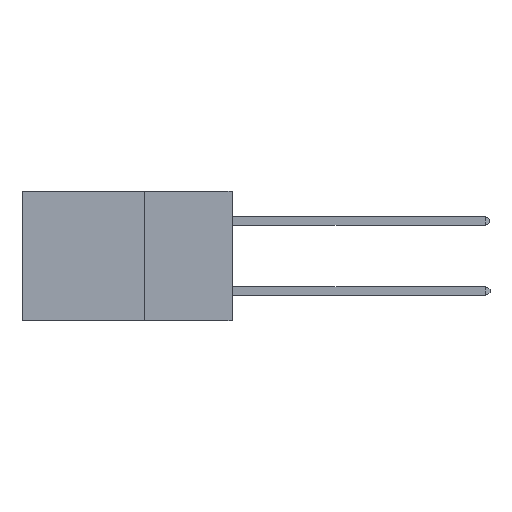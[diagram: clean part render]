
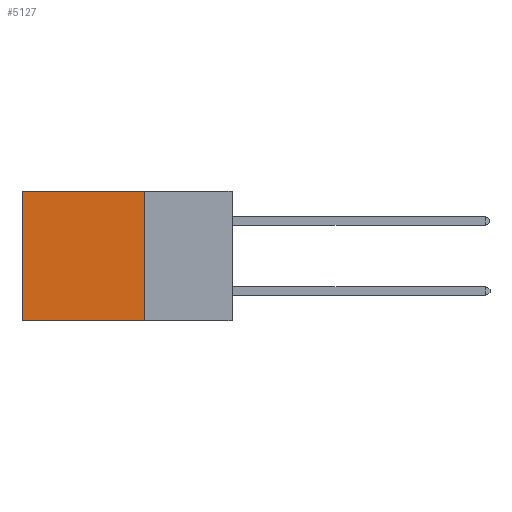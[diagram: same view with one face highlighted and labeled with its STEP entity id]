
A CAD part, left-side view. The second image highlights one B-rep face of the part: STEP entity #5127.
In plain terms, the highlighted planar face has unit normal (-1, 0, 0).
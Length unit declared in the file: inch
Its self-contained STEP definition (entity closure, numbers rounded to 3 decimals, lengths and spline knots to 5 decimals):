
#212 = EDGE_CURVE ( 'NONE', #12373, #5416, #5501, .T. ) ;
#460 = CARTESIAN_POINT ( 'NONE',  ( 0.2875, 0.6, -0.37 ) ) ;
#542 = FACE_OUTER_BOUND ( 'NONE', #8381, .T. ) ;
#836 = LINE ( 'NONE', #8320, #11488 ) ;
#1406 = VECTOR ( 'NONE', #11920, 39.37008 ) ;
#1836 = LINE ( 'NONE', #11827, #1406 ) ;
#2302 = EDGE_CURVE ( 'NONE', #6231, #5416, #6464, .T. ) ;
#2935 = EDGE_CURVE ( 'NONE', #16811, #12373, #836, .T. ) ;
#3897 = ORIENTED_EDGE ( 'NONE', *, *, #212, .F. ) ;
#4530 = EDGE_CURVE ( 'NONE', #16811, #6231, #1836, .T. ) ;
#4585 = DIRECTION ( 'NONE',  ( 0., 0., -1. ) ) ;
#4605 = DIRECTION ( 'NONE',  ( 1., 0., 0. ) ) ;
#4776 = AXIS2_PLACEMENT_3D ( 'NONE', #4780, #4605, #4585 ) ;
#4780 = CARTESIAN_POINT ( 'NONE',  ( 0.2875, 0.25, 0. ) ) ;
#4921 = PLANE ( 'NONE',  #4776 ) ;
#4970 = DIRECTION ( 'NONE',  ( 0., 1., 0. ) ) ;
#5127 = ADVANCED_FACE ( 'NONE', ( #542 ), #4921, .F. ) ;
#5416 = VERTEX_POINT ( 'NONE', #460 ) ;
#5501 = LINE ( 'NONE', #11402, #15420 ) ;
#6184 = ORIENTED_EDGE ( 'NONE', *, *, #2302, .T. ) ;
#6231 = VERTEX_POINT ( 'NONE', #13416 ) ;
#6464 = LINE ( 'NONE', #16905, #9092 ) ;
#8293 = DIRECTION ( 'NONE',  ( 0., 0., -1. ) ) ;
#8307 = ORIENTED_EDGE ( 'NONE', *, *, #2935, .F. ) ;
#8320 = CARTESIAN_POINT ( 'NONE',  ( 0.2875, 0.25, 0. ) ) ;
#8381 = EDGE_LOOP ( 'NONE', ( #6184, #3897, #8307, #12264 ) ) ;
#8444 = CARTESIAN_POINT ( 'NONE',  ( 0.2875, 0.25, 0. ) ) ;
#9092 = VECTOR ( 'NONE', #16817, 39.37008 ) ;
#10881 = CARTESIAN_POINT ( 'NONE',  ( 0.2875, 0.25, -0.37 ) ) ;
#11402 = CARTESIAN_POINT ( 'NONE',  ( 0.2875, 0.25, -0.37 ) ) ;
#11488 = VECTOR ( 'NONE', #8293, 39.37008 ) ;
#11827 = CARTESIAN_POINT ( 'NONE',  ( 0.2875, 0.25, 0. ) ) ;
#11920 = DIRECTION ( 'NONE',  ( 0., 1., 0. ) ) ;
#12264 = ORIENTED_EDGE ( 'NONE', *, *, #4530, .T. ) ;
#12373 = VERTEX_POINT ( 'NONE', #10881 ) ;
#13416 = CARTESIAN_POINT ( 'NONE',  ( 0.2875, 0.6, 0. ) ) ;
#15420 = VECTOR ( 'NONE', #4970, 39.37008 ) ;
#16811 = VERTEX_POINT ( 'NONE', #8444 ) ;
#16817 = DIRECTION ( 'NONE',  ( 0., 0., -1. ) ) ;
#16905 = CARTESIAN_POINT ( 'NONE',  ( 0.2875, 0.6, 0. ) ) ;
